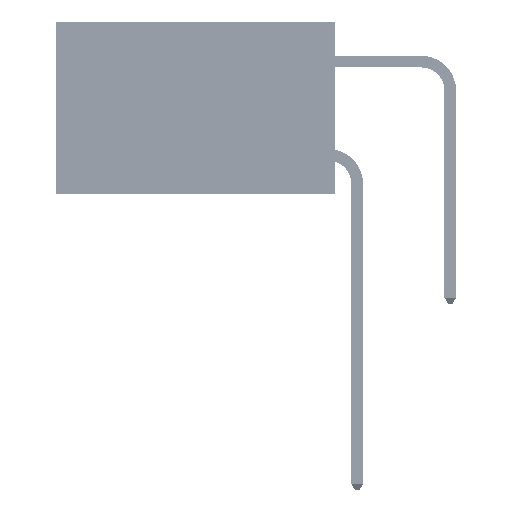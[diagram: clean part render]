
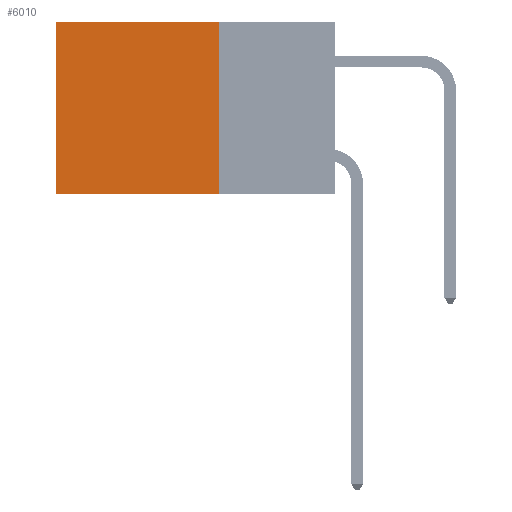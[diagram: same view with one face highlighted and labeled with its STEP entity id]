
A CAD part, left-side view. The second image highlights one B-rep face of the part: STEP entity #6010.
In plain terms, the highlighted planar face has unit normal (-1, 0, 0).
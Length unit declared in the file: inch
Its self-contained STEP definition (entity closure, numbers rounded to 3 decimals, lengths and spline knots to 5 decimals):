
#1586 = ORIENTED_EDGE ( 'NONE', *, *, #6188, .F. ) ;
#2903 = CARTESIAN_POINT ( 'NONE',  ( 0.2875, 0.25, 0. ) ) ;
#3255 = DIRECTION ( 'NONE',  ( 0., 1., 0. ) ) ;
#3616 = EDGE_CURVE ( 'NONE', #44248, #9020, #33753, .T. ) ;
#4597 = DIRECTION ( 'NONE',  ( 0., 0., -1. ) ) ;
#4655 = VECTOR ( 'NONE', #4597, 39.37008 ) ;
#5261 = EDGE_CURVE ( 'NONE', #44248, #31969, #36170, .T. ) ;
#6010 = ADVANCED_FACE ( 'NONE', ( #31569 ), #6759, .F. ) ;
#6188 = EDGE_CURVE ( 'NONE', #31969, #20011, #16600, .T. ) ;
#6759 = PLANE ( 'NONE',  #49834 ) ;
#9020 = VERTEX_POINT ( 'NONE', #22618 ) ;
#16133 = CARTESIAN_POINT ( 'NONE',  ( 0.2875, 0.25, 0. ) ) ;
#16600 = LINE ( 'NONE', #20041, #34102 ) ;
#16733 = DIRECTION ( 'NONE',  ( 0., 1., 0. ) ) ;
#19346 = DIRECTION ( 'NONE',  ( 0., 0., -1. ) ) ;
#19503 = ORIENTED_EDGE ( 'NONE', *, *, #20464, .T. ) ;
#19566 = VECTOR ( 'NONE', #3255, 39.37008 ) ;
#19995 = DIRECTION ( 'NONE',  ( 0., 0., -1. ) ) ;
#20011 = VERTEX_POINT ( 'NONE', #30865 ) ;
#20041 = CARTESIAN_POINT ( 'NONE',  ( 0.2875, 0.25, -0.37 ) ) ;
#20464 = EDGE_CURVE ( 'NONE', #9020, #20011, #26671, .T. ) ;
#20884 = CARTESIAN_POINT ( 'NONE',  ( 0.2875, 0.25, 0. ) ) ;
#22618 = CARTESIAN_POINT ( 'NONE',  ( 0.2875, 0.6, 0. ) ) ;
#23183 = CARTESIAN_POINT ( 'NONE',  ( 0.2875, 0.25, 0. ) ) ;
#25627 = CARTESIAN_POINT ( 'NONE',  ( 0.2875, 0.6, 0. ) ) ;
#25689 = ORIENTED_EDGE ( 'NONE', *, *, #5261, .F. ) ;
#26671 = LINE ( 'NONE', #25627, #4655 ) ;
#27114 = VECTOR ( 'NONE', #19346, 39.37008 ) ;
#30865 = CARTESIAN_POINT ( 'NONE',  ( 0.2875, 0.6, -0.37 ) ) ;
#31569 = FACE_OUTER_BOUND ( 'NONE', #41460, .T. ) ;
#31969 = VERTEX_POINT ( 'NONE', #47778 ) ;
#33753 = LINE ( 'NONE', #2903, #19566 ) ;
#34102 = VECTOR ( 'NONE', #16733, 39.37008 ) ;
#36170 = LINE ( 'NONE', #23183, #27114 ) ;
#41460 = EDGE_LOOP ( 'NONE', ( #19503, #1586, #25689, #44491 ) ) ;
#44248 = VERTEX_POINT ( 'NONE', #20884 ) ;
#44491 = ORIENTED_EDGE ( 'NONE', *, *, #3616, .T. ) ;
#47778 = CARTESIAN_POINT ( 'NONE',  ( 0.2875, 0.25, -0.37 ) ) ;
#49300 = DIRECTION ( 'NONE',  ( 1., 0., 0. ) ) ;
#49834 = AXIS2_PLACEMENT_3D ( 'NONE', #16133, #49300, #19995 ) ;
